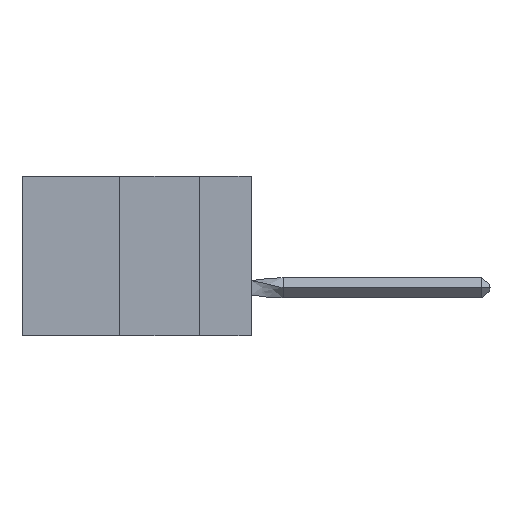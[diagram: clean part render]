
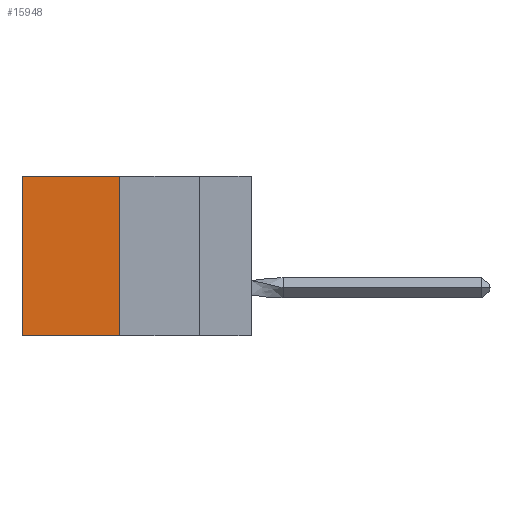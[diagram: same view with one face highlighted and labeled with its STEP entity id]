
A CAD part, left-side view. The second image highlights one B-rep face of the part: STEP entity #15948.
In plain terms, the highlighted planar face has unit normal (-1, 0, 0).
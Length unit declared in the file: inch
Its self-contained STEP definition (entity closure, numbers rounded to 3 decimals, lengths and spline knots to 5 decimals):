
#371 = FACE_OUTER_BOUND ( 'NONE', #13094, .T. ) ;
#1040 = ORIENTED_EDGE ( 'NONE', *, *, #32031, .F. ) ;
#1458 = CARTESIAN_POINT ( 'NONE',  ( 0.305, 0.72, -0.5 ) ) ;
#2238 = DIRECTION ( 'NONE',  ( 1., 0., 0. ) ) ;
#3360 = LINE ( 'NONE', #1458, #4520 ) ;
#4112 = CARTESIAN_POINT ( 'NONE',  ( 0.305, 0.413, -0.5 ) ) ;
#4520 = VECTOR ( 'NONE', #26565, 39.37008 ) ;
#6185 = VECTOR ( 'NONE', #14272, 39.37008 ) ;
#7630 = PLANE ( 'NONE',  #25511 ) ;
#8422 = CARTESIAN_POINT ( 'NONE',  ( 0.305, 0.413, -0.5 ) ) ;
#8532 = DIRECTION ( 'NONE',  ( 0., 0., -1. ) ) ;
#8705 = CARTESIAN_POINT ( 'NONE',  ( 0.305, 0.413, 0. ) ) ;
#9738 = CARTESIAN_POINT ( 'NONE',  ( 0.305, 0.413, -0.5 ) ) ;
#10578 = VERTEX_POINT ( 'NONE', #29227 ) ;
#10633 = LINE ( 'NONE', #8705, #16138 ) ;
#12626 = VERTEX_POINT ( 'NONE', #16936 ) ;
#12643 = VECTOR ( 'NONE', #8532, 39.37008 ) ;
#13094 = EDGE_LOOP ( 'NONE', ( #15876, #15644, #1040, #24240 ) ) ;
#14272 = DIRECTION ( 'NONE',  ( 0., 1., 0. ) ) ;
#15020 = LINE ( 'NONE', #23456, #12643 ) ;
#15644 = ORIENTED_EDGE ( 'NONE', *, *, #17267, .F. ) ;
#15876 = ORIENTED_EDGE ( 'NONE', *, *, #19364, .T. ) ;
#15948 = ADVANCED_FACE ( 'NONE', ( #371 ), #7630, .F. ) ;
#16072 = LINE ( 'NONE', #8422, #6185 ) ;
#16138 = VECTOR ( 'NONE', #19062, 39.37008 ) ;
#16936 = CARTESIAN_POINT ( 'NONE',  ( 0.305, 0.413, 0. ) ) ;
#17267 = EDGE_CURVE ( 'NONE', #23931, #10578, #16072, .T. ) ;
#19062 = DIRECTION ( 'NONE',  ( 0., 1., 0. ) ) ;
#19364 = EDGE_CURVE ( 'NONE', #25491, #10578, #3360, .T. ) ;
#19738 = CARTESIAN_POINT ( 'NONE',  ( 0.305, 0.72, 0. ) ) ;
#22447 = DIRECTION ( 'NONE',  ( 0., 0., -1. ) ) ;
#23456 = CARTESIAN_POINT ( 'NONE',  ( 0.305, 0.413, -0.5 ) ) ;
#23931 = VERTEX_POINT ( 'NONE', #4112 ) ;
#24240 = ORIENTED_EDGE ( 'NONE', *, *, #32685, .T. ) ;
#25491 = VERTEX_POINT ( 'NONE', #19738 ) ;
#25511 = AXIS2_PLACEMENT_3D ( 'NONE', #9738, #2238, #22447 ) ;
#26565 = DIRECTION ( 'NONE',  ( 0., 0., -1. ) ) ;
#29227 = CARTESIAN_POINT ( 'NONE',  ( 0.305, 0.72, -0.5 ) ) ;
#32031 = EDGE_CURVE ( 'NONE', #12626, #23931, #15020, .T. ) ;
#32685 = EDGE_CURVE ( 'NONE', #12626, #25491, #10633, .T. ) ;
